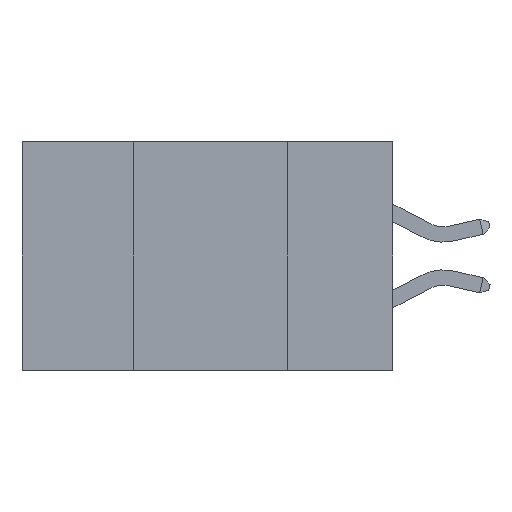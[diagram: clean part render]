
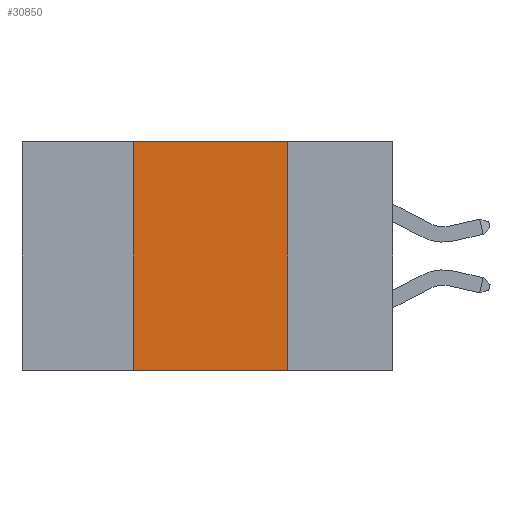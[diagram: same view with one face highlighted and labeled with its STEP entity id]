
A CAD part, left-side view. The second image highlights one B-rep face of the part: STEP entity #30850.
In plain terms, the highlighted planar face has unit normal (-1, 0, 0).
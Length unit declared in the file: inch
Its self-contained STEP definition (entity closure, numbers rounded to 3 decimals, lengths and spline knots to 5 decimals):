
#912 = EDGE_CURVE ( 'NONE', #21484, #41131, #25346, .T. ) ;
#1285 = DIRECTION ( 'NONE',  ( 0., -1., 0. ) ) ;
#2481 = DIRECTION ( 'NONE',  ( 0., -1., 0. ) ) ;
#6427 = VECTOR ( 'NONE', #2481, 39.37008 ) ;
#6504 = CARTESIAN_POINT ( 'NONE',  ( 0., 0.17, -0.37 ) ) ;
#7850 = CARTESIAN_POINT ( 'NONE',  ( 0., 0.6, -0.37 ) ) ;
#8604 = DIRECTION ( 'NONE',  ( 0., 0., -1. ) ) ;
#8990 = VECTOR ( 'NONE', #1285, 39.37008 ) ;
#10514 = LINE ( 'NONE', #7850, #8990 ) ;
#13875 = CARTESIAN_POINT ( 'NONE',  ( 0., 0.42, 0. ) ) ;
#14946 = ORIENTED_EDGE ( 'NONE', *, *, #912, .F. ) ;
#14999 = CARTESIAN_POINT ( 'NONE',  ( 0., 0.42, 0. ) ) ;
#15046 = DIRECTION ( 'NONE',  ( 1., 0., 0. ) ) ;
#15411 = CARTESIAN_POINT ( 'NONE',  ( 0., 0.6, 0. ) ) ;
#20563 = CARTESIAN_POINT ( 'NONE',  ( 0., 0.42, -0.37 ) ) ;
#20845 = DIRECTION ( 'NONE',  ( 0., 0., 1. ) ) ;
#21144 = FACE_OUTER_BOUND ( 'NONE', #25148, .T. ) ;
#21302 = EDGE_CURVE ( 'NONE', #38559, #21484, #25871, .T. ) ;
#21312 = EDGE_CURVE ( 'NONE', #38559, #37198, #10514, .T. ) ;
#21484 = VERTEX_POINT ( 'NONE', #14999 ) ;
#22116 = AXIS2_PLACEMENT_3D ( 'NONE', #31481, #15046, #8604 ) ;
#23878 = EDGE_CURVE ( 'NONE', #41131, #37198, #34162, .T. ) ;
#25148 = EDGE_LOOP ( 'NONE', ( #34624, #14946, #28286, #32070 ) ) ;
#25346 = LINE ( 'NONE', #15411, #6427 ) ;
#25495 = VECTOR ( 'NONE', #37502, 39.37008 ) ;
#25871 = LINE ( 'NONE', #13875, #41172 ) ;
#28286 = ORIENTED_EDGE ( 'NONE', *, *, #21302, .F. ) ;
#30850 = ADVANCED_FACE ( 'NONE', ( #21144 ), #41307, .F. ) ;
#31481 = CARTESIAN_POINT ( 'NONE',  ( 0., 0.6, 0. ) ) ;
#32070 = ORIENTED_EDGE ( 'NONE', *, *, #21312, .T. ) ;
#33962 = CARTESIAN_POINT ( 'NONE',  ( 0., 0.17, 0. ) ) ;
#34162 = LINE ( 'NONE', #33962, #25495 ) ;
#34624 = ORIENTED_EDGE ( 'NONE', *, *, #23878, .F. ) ;
#37198 = VERTEX_POINT ( 'NONE', #6504 ) ;
#37502 = DIRECTION ( 'NONE',  ( 0., 0., -1. ) ) ;
#38559 = VERTEX_POINT ( 'NONE', #20563 ) ;
#41131 = VERTEX_POINT ( 'NONE', #41552 ) ;
#41172 = VECTOR ( 'NONE', #20845, 39.37008 ) ;
#41307 = PLANE ( 'NONE',  #22116 ) ;
#41552 = CARTESIAN_POINT ( 'NONE',  ( 0., 0.17, 0. ) ) ;
